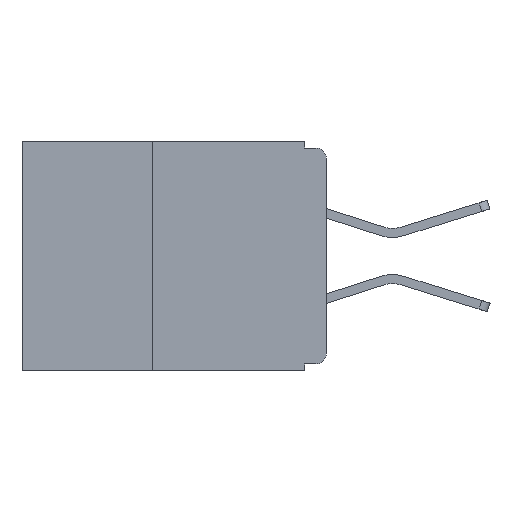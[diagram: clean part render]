
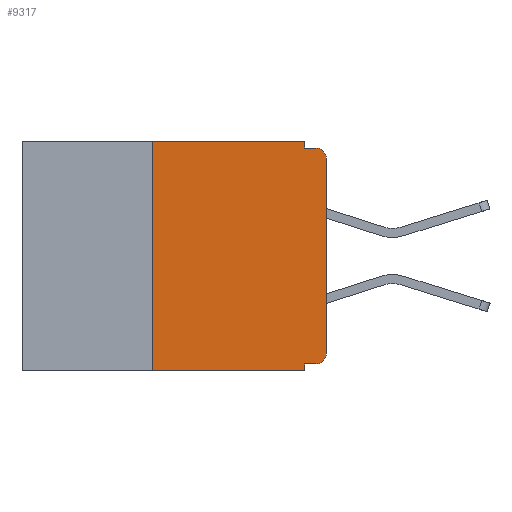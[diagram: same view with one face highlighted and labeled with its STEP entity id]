
A CAD part, left-side view. The second image highlights one B-rep face of the part: STEP entity #9317.
In plain terms, the highlighted planar face has unit normal (-1, 0, 0).
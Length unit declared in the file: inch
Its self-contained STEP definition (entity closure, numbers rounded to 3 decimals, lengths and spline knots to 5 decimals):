
#516 = ORIENTED_EDGE ( 'NONE', *, *, #8438, .T. ) ;
#587 = ORIENTED_EDGE ( 'NONE', *, *, #2564, .T. ) ;
#603 = ORIENTED_EDGE ( 'NONE', *, *, #2350, .F. ) ;
#632 = ORIENTED_EDGE ( 'NONE', *, *, #1721, .F. ) ;
#671 = ORIENTED_EDGE ( 'NONE', *, *, #973, .F. ) ;
#710 = ORIENTED_EDGE ( 'NONE', *, *, #1723, .F. ) ;
#776 = CARTESIAN_POINT ( 'NONE',  ( 0., 0.031, -0.01 ) ) ;
#865 = ORIENTED_EDGE ( 'NONE', *, *, #1752, .T. ) ;
#905 = EDGE_LOOP ( 'NONE', ( #516, #587, #603, #632, #671, #710, #865, #974, #1001, #1071 ) ) ;
#935 = CARTESIAN_POINT ( 'NONE',  ( 0., 0.25, -0.33 ) ) ;
#973 = EDGE_CURVE ( 'NONE', #11799, #6332, #5278, .T. ) ;
#974 = ORIENTED_EDGE ( 'NONE', *, *, #1785, .F. ) ;
#1001 = ORIENTED_EDGE ( 'NONE', *, *, #4902, .F. ) ;
#1071 = ORIENTED_EDGE ( 'NONE', *, *, #10706, .T. ) ;
#1148 = CARTESIAN_POINT ( 'NONE',  ( 0., 0.015, -0.32 ) ) ;
#1476 = CARTESIAN_POINT ( 'NONE',  ( 0., 0., -0.305 ) ) ;
#1607 = FACE_OUTER_BOUND ( 'NONE', #905, .T. ) ;
#1677 = VERTEX_POINT ( 'NONE', #6345 ) ;
#1721 = EDGE_CURVE ( 'NONE', #6332, #10783, #4530, .T. ) ;
#1723 = EDGE_CURVE ( 'NONE', #10237, #11799, #4407, .T. ) ;
#1752 = EDGE_CURVE ( 'NONE', #10237, #1677, #3397, .T. ) ;
#1785 = EDGE_CURVE ( 'NONE', #11832, #1677, #3183, .T. ) ;
#1957 = CARTESIAN_POINT ( 'NONE',  ( 0., 0.031, 0. ) ) ;
#2097 = VECTOR ( 'NONE', #2103, 39.37008 ) ;
#2103 = DIRECTION ( 'NONE',  ( 0., 0., -1. ) ) ;
#2345 = CARTESIAN_POINT ( 'NONE',  ( 0., 0.031, -0.33 ) ) ;
#2350 = EDGE_CURVE ( 'NONE', #10783, #2526, #6193, .T. ) ;
#2526 = VERTEX_POINT ( 'NONE', #6562 ) ;
#2564 = EDGE_CURVE ( 'NONE', #5578, #2526, #11587, .T. ) ;
#2860 = CIRCLE ( 'NONE', #5129, 0.015 ) ;
#2886 = VECTOR ( 'NONE', #11185, 39.37008 ) ;
#3183 = LINE ( 'NONE', #2345, #2097 ) ;
#3189 = CARTESIAN_POINT ( 'NONE',  ( 0., 0., -0.025 ) ) ;
#3200 = DIRECTION ( 'NONE',  ( 0., -1., 0. ) ) ;
#3220 = CARTESIAN_POINT ( 'NONE',  ( 0., 0.031, -0.32 ) ) ;
#3230 = VECTOR ( 'NONE', #5290, 39.37008 ) ;
#3241 = LINE ( 'NONE', #6427, #3230 ) ;
#3397 = LINE ( 'NONE', #9759, #2886 ) ;
#3448 = CARTESIAN_POINT ( 'NONE',  ( 0., 0.25, 0. ) ) ;
#3748 = VERTEX_POINT ( 'NONE', #1476 ) ;
#4094 = VECTOR ( 'NONE', #10059, 39.37008 ) ;
#4348 = VECTOR ( 'NONE', #10153, 39.37008 ) ;
#4407 = LINE ( 'NONE', #935, #4094 ) ;
#4530 = LINE ( 'NONE', #1957, #4348 ) ;
#4902 = EDGE_CURVE ( 'NONE', #6203, #11832, #10437, .T. ) ;
#4984 = VECTOR ( 'NONE', #3200, 39.37008 ) ;
#5129 = AXIS2_PLACEMENT_3D ( 'NONE', #5339, #5247, #5229 ) ;
#5133 = VECTOR ( 'NONE', #8328, 39.37008 ) ;
#5229 = DIRECTION ( 'NONE',  ( 0., 0., -1. ) ) ;
#5247 = DIRECTION ( 'NONE',  ( -1., 0., 0. ) ) ;
#5278 = LINE ( 'NONE', #8566, #5133 ) ;
#5290 = DIRECTION ( 'NONE',  ( 0., 0., 1. ) ) ;
#5296 = AXIS2_PLACEMENT_3D ( 'NONE', #7862, #7353, #7334 ) ;
#5339 = CARTESIAN_POINT ( 'NONE',  ( 0., 0.015, -0.305 ) ) ;
#5443 = DIRECTION ( 'NONE',  ( 0., 1., 0. ) ) ;
#5578 = VERTEX_POINT ( 'NONE', #3189 ) ;
#5834 = CARTESIAN_POINT ( 'NONE',  ( 0., 0., -0.32 ) ) ;
#5942 = CARTESIAN_POINT ( 'NONE',  ( 0., 0.25, -0.33 ) ) ;
#6193 = LINE ( 'NONE', #8419, #4984 ) ;
#6203 = VERTEX_POINT ( 'NONE', #1148 ) ;
#6332 = VERTEX_POINT ( 'NONE', #9292 ) ;
#6345 = CARTESIAN_POINT ( 'NONE',  ( 0., 0.031, -0.33 ) ) ;
#6427 = CARTESIAN_POINT ( 'NONE',  ( 0., 0., 0. ) ) ;
#6562 = CARTESIAN_POINT ( 'NONE',  ( 0., 0.015, -0.01 ) ) ;
#7334 = DIRECTION ( 'NONE',  ( 0., 0., -1. ) ) ;
#7353 = DIRECTION ( 'NONE',  ( 1., 0., 0. ) ) ;
#7509 = DIRECTION ( 'NONE',  ( 0., 0., -1. ) ) ;
#7513 = DIRECTION ( 'NONE',  ( -1., 0., 0. ) ) ;
#7524 = CARTESIAN_POINT ( 'NONE',  ( 0., 0.015, -0.025 ) ) ;
#7862 = CARTESIAN_POINT ( 'NONE',  ( 0., 0.437, 0. ) ) ;
#8304 = PLANE ( 'NONE',  #5296 ) ;
#8328 = DIRECTION ( 'NONE',  ( 0., -1., 0. ) ) ;
#8419 = CARTESIAN_POINT ( 'NONE',  ( 0., 0., -0.01 ) ) ;
#8438 = EDGE_CURVE ( 'NONE', #3748, #5578, #3241, .T. ) ;
#8566 = CARTESIAN_POINT ( 'NONE',  ( 0., 0.437, 0. ) ) ;
#9292 = CARTESIAN_POINT ( 'NONE',  ( 0., 0.031, 0. ) ) ;
#9317 = ADVANCED_FACE ( 'NONE', ( #1607 ), #8304, .F. ) ;
#9759 = CARTESIAN_POINT ( 'NONE',  ( 0., 0.437, -0.33 ) ) ;
#10059 = DIRECTION ( 'NONE',  ( 0., 0., 1. ) ) ;
#10153 = DIRECTION ( 'NONE',  ( 0., 0., -1. ) ) ;
#10237 = VERTEX_POINT ( 'NONE', #5942 ) ;
#10437 = LINE ( 'NONE', #5834, #10970 ) ;
#10706 = EDGE_CURVE ( 'NONE', #6203, #3748, #2860, .T. ) ;
#10783 = VERTEX_POINT ( 'NONE', #776 ) ;
#10970 = VECTOR ( 'NONE', #5443, 39.37008 ) ;
#11185 = DIRECTION ( 'NONE',  ( 0., -1., 0. ) ) ;
#11587 = CIRCLE ( 'NONE', #11742, 0.015 ) ;
#11742 = AXIS2_PLACEMENT_3D ( 'NONE', #7524, #7513, #7509 ) ;
#11799 = VERTEX_POINT ( 'NONE', #3448 ) ;
#11832 = VERTEX_POINT ( 'NONE', #3220 ) ;
